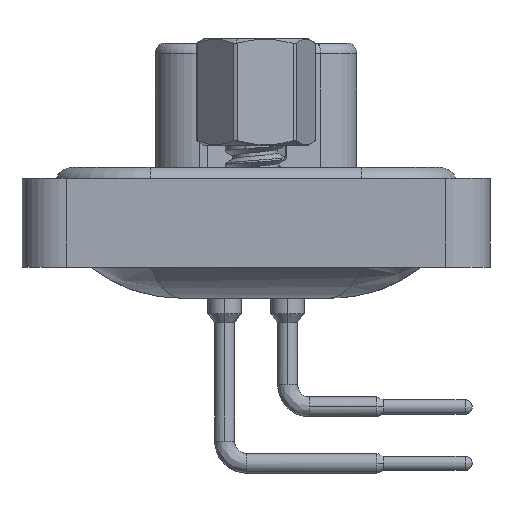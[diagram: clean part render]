
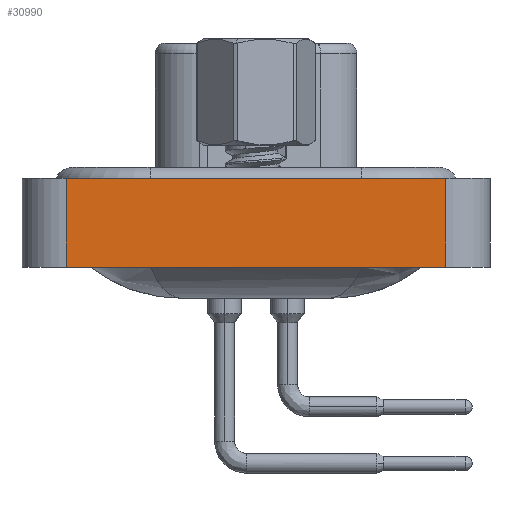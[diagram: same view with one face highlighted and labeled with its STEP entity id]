
A CAD part, left-side view. The second image highlights one B-rep face of the part: STEP entity #30990.
In plain terms, the highlighted planar face has unit normal (-1, 0, 0).
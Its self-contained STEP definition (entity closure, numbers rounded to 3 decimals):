
#1770 = FACE_OUTER_BOUND ( 'NONE', #28720, .T. ) ;
#2170 = LINE ( 'NONE', #12314, #31336 ) ;
#2336 = DIRECTION ( 'NONE',  ( 0., 0., 1. ) ) ;
#3294 = EDGE_CURVE ( 'NONE', #15145, #26631, #22681, .T. ) ;
#3405 = ORIENTED_EDGE ( 'NONE', *, *, #3294, .T. ) ;
#3989 = EDGE_CURVE ( 'NONE', #26631, #20425, #15974, .T. ) ;
#4309 = ORIENTED_EDGE ( 'NONE', *, *, #24771, .F. ) ;
#4554 = ORIENTED_EDGE ( 'NONE', *, *, #30129, .F. ) ;
#4735 = DIRECTION ( 'NONE',  ( 0., -1., 0. ) ) ;
#4910 = VECTOR ( 'NONE', #21254, 1000. ) ;
#9402 = CARTESIAN_POINT ( 'NONE',  ( -7.35, -8.55, -3.6 ) ) ;
#10903 = LINE ( 'NONE', #21016, #15278 ) ;
#12314 = CARTESIAN_POINT ( 'NONE',  ( -7.35, 8.55, -3.6 ) ) ;
#15145 = VERTEX_POINT ( 'NONE', #18709 ) ;
#15278 = VECTOR ( 'NONE', #24009, 1000. ) ;
#15438 = VERTEX_POINT ( 'NONE', #23000 ) ;
#15974 = LINE ( 'NONE', #28896, #4910 ) ;
#18709 = CARTESIAN_POINT ( 'NONE',  ( -7.35, 8.55, -3.6 ) ) ;
#18773 = CARTESIAN_POINT ( 'NONE',  ( -7.35, -8.55, -3.6 ) ) ;
#19527 = DIRECTION ( 'NONE',  ( -1., 0., 0. ) ) ;
#20253 = VECTOR ( 'NONE', #4735, 1000. ) ;
#20425 = VERTEX_POINT ( 'NONE', #31520 ) ;
#21016 = CARTESIAN_POINT ( 'NONE',  ( -7.35, -8.55, 0.4 ) ) ;
#21254 = DIRECTION ( 'NONE',  ( 0., 0., 1. ) ) ;
#21658 = ORIENTED_EDGE ( 'NONE', *, *, #3989, .T. ) ;
#22028 = PLANE ( 'NONE',  #24322 ) ;
#22681 = LINE ( 'NONE', #25020, #20253 ) ;
#23000 = CARTESIAN_POINT ( 'NONE',  ( -7.35, 8.55, 0.4 ) ) ;
#23861 = DIRECTION ( 'NONE',  ( 0., 0., 1. ) ) ;
#24009 = DIRECTION ( 'NONE',  ( 0., -1., 0. ) ) ;
#24322 = AXIS2_PLACEMENT_3D ( 'NONE', #9402, #19527, #23861 ) ;
#24771 = EDGE_CURVE ( 'NONE', #15145, #15438, #2170, .T. ) ;
#25020 = CARTESIAN_POINT ( 'NONE',  ( -7.35, -8.55, -3.6 ) ) ;
#26631 = VERTEX_POINT ( 'NONE', #18773 ) ;
#28720 = EDGE_LOOP ( 'NONE', ( #21658, #4554, #4309, #3405 ) ) ;
#28896 = CARTESIAN_POINT ( 'NONE',  ( -7.35, -8.55, -3.6 ) ) ;
#30129 = EDGE_CURVE ( 'NONE', #15438, #20425, #10903, .T. ) ;
#30990 = ADVANCED_FACE ( 'NONE', ( #1770 ), #22028, .T. ) ;
#31336 = VECTOR ( 'NONE', #2336, 1000. ) ;
#31520 = CARTESIAN_POINT ( 'NONE',  ( -7.35, -8.55, 0.4 ) ) ;
